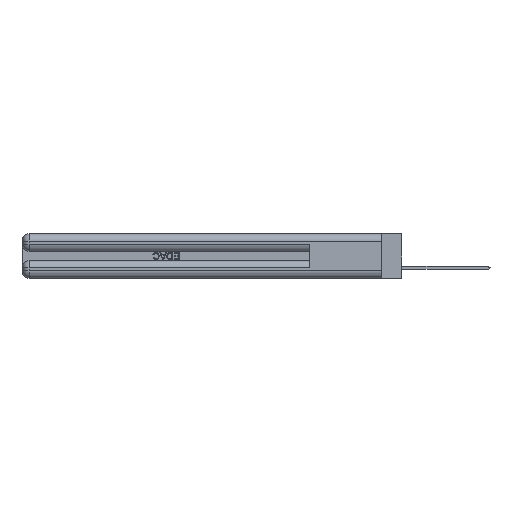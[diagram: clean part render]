
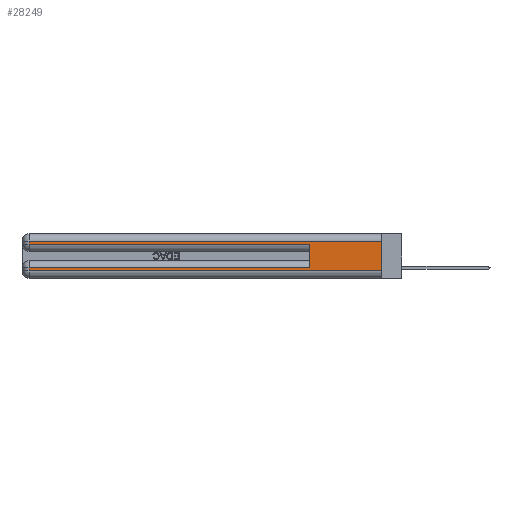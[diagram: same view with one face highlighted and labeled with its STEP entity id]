
A CAD part, left-side view. The second image highlights one B-rep face of the part: STEP entity #28249.
In plain terms, the highlighted planar face has unit normal (-1, 0, 0).
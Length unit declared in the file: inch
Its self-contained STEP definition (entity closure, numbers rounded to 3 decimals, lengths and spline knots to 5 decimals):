
#190 = LINE ( 'NONE', #8576, #42534 ) ;
#1328 = PLANE ( 'NONE',  #21933 ) ;
#1861 = DIRECTION ( 'NONE',  ( 0., 0., -1. ) ) ;
#3652 = CARTESIAN_POINT ( 'NONE',  ( 0., 2.94, 0.37 ) ) ;
#4363 = VECTOR ( 'NONE', #33084, 39.37008 ) ;
#4676 = VERTEX_POINT ( 'NONE', #18615 ) ;
#5362 = CARTESIAN_POINT ( 'NONE',  ( 0., 2.94, 0.37 ) ) ;
#5512 = CARTESIAN_POINT ( 'NONE',  ( 0., 0., 0.37 ) ) ;
#6326 = ORIENTED_EDGE ( 'NONE', *, *, #7794, .T. ) ;
#7229 = LINE ( 'NONE', #30174, #17976 ) ;
#7293 = DIRECTION ( 'NONE',  ( 0., -1., 0. ) ) ;
#7794 = EDGE_CURVE ( 'NONE', #32536, #46410, #32329, .T. ) ;
#8022 = EDGE_CURVE ( 'NONE', #26386, #9400, #7229, .T. ) ;
#8324 = EDGE_CURVE ( 'NONE', #19796, #9400, #21533, .T. ) ;
#8576 = CARTESIAN_POINT ( 'NONE',  ( 0., 0., 0.06 ) ) ;
#9400 = VERTEX_POINT ( 'NONE', #36453 ) ;
#9768 = ORIENTED_EDGE ( 'NONE', *, *, #26087, .T. ) ;
#9895 = VECTOR ( 'NONE', #1861, 39.37008 ) ;
#9980 = EDGE_LOOP ( 'NONE', ( #30056, #23095, #9768, #12261, #47401, #27262, #6326, #43001 ) ) ;
#10541 = CARTESIAN_POINT ( 'NONE',  ( 0., 0., 0.37 ) ) ;
#10996 = CARTESIAN_POINT ( 'NONE',  ( 0., 2.94, 0.06 ) ) ;
#12261 = ORIENTED_EDGE ( 'NONE', *, *, #8022, .T. ) ;
#13744 = CARTESIAN_POINT ( 'NONE',  ( 0., 0.6, 0.085 ) ) ;
#14297 = EDGE_CURVE ( 'NONE', #19796, #32536, #23885, .T. ) ;
#14438 = LINE ( 'NONE', #39794, #23378 ) ;
#17976 = VECTOR ( 'NONE', #7293, 39.37008 ) ;
#18615 = CARTESIAN_POINT ( 'NONE',  ( 0., 0., 0.06 ) ) ;
#19615 = CARTESIAN_POINT ( 'NONE',  ( 0., 0., 0.085 ) ) ;
#19714 = VECTOR ( 'NONE', #23392, 39.37008 ) ;
#19728 = VECTOR ( 'NONE', #23455, 39.37008 ) ;
#19796 = VERTEX_POINT ( 'NONE', #13744 ) ;
#21533 = LINE ( 'NONE', #46171, #19714 ) ;
#21619 = DIRECTION ( 'NONE',  ( 0., 1., 0. ) ) ;
#21933 = AXIS2_PLACEMENT_3D ( 'NONE', #5512, #31906, #39918 ) ;
#22198 = VECTOR ( 'NONE', #45498, 39.37008 ) ;
#23095 = ORIENTED_EDGE ( 'NONE', *, *, #29422, .T. ) ;
#23378 = VECTOR ( 'NONE', #21619, 39.37008 ) ;
#23392 = DIRECTION ( 'NONE',  ( 0., 0., 1. ) ) ;
#23455 = DIRECTION ( 'NONE',  ( 0., 1., 0. ) ) ;
#23595 = VERTEX_POINT ( 'NONE', #43406 ) ;
#23885 = LINE ( 'NONE', #19615, #19728 ) ;
#26087 = EDGE_CURVE ( 'NONE', #23595, #26386, #48061, .T. ) ;
#26386 = VERTEX_POINT ( 'NONE', #39602 ) ;
#27262 = ORIENTED_EDGE ( 'NONE', *, *, #14297, .T. ) ;
#28249 = ADVANCED_FACE ( 'NONE', ( #37315 ), #1328, .F. ) ;
#29422 = EDGE_CURVE ( 'NONE', #48343, #23595, #14438, .T. ) ;
#30056 = ORIENTED_EDGE ( 'NONE', *, *, #42595, .F. ) ;
#30174 = CARTESIAN_POINT ( 'NONE',  ( 0., 0., 0.285 ) ) ;
#30803 = CARTESIAN_POINT ( 'NONE',  ( 0., 2.94, 0.085 ) ) ;
#31906 = DIRECTION ( 'NONE',  ( 1., 0., 0. ) ) ;
#32329 = LINE ( 'NONE', #3652, #22198 ) ;
#32536 = VERTEX_POINT ( 'NONE', #30803 ) ;
#33084 = DIRECTION ( 'NONE',  ( 0., 0., -1. ) ) ;
#36453 = CARTESIAN_POINT ( 'NONE',  ( 0., 0.6, 0.285 ) ) ;
#37315 = FACE_OUTER_BOUND ( 'NONE', #9980, .T. ) ;
#38466 = CARTESIAN_POINT ( 'NONE',  ( 0., 0., 0.31 ) ) ;
#39602 = CARTESIAN_POINT ( 'NONE',  ( 0., 2.94, 0.285 ) ) ;
#39794 = CARTESIAN_POINT ( 'NONE',  ( 0., 0., 0.31 ) ) ;
#39918 = DIRECTION ( 'NONE',  ( 0., 0., -1. ) ) ;
#42534 = VECTOR ( 'NONE', #47076, 39.37008 ) ;
#42595 = EDGE_CURVE ( 'NONE', #48343, #4676, #44990, .T. ) ;
#43001 = ORIENTED_EDGE ( 'NONE', *, *, #47907, .T. ) ;
#43406 = CARTESIAN_POINT ( 'NONE',  ( 0., 2.94, 0.31 ) ) ;
#44990 = LINE ( 'NONE', #10541, #4363 ) ;
#45498 = DIRECTION ( 'NONE',  ( 0., 0., -1. ) ) ;
#46171 = CARTESIAN_POINT ( 'NONE',  ( 0., 0.6, 0.145 ) ) ;
#46410 = VERTEX_POINT ( 'NONE', #10996 ) ;
#47076 = DIRECTION ( 'NONE',  ( 0., -1., 0. ) ) ;
#47401 = ORIENTED_EDGE ( 'NONE', *, *, #8324, .F. ) ;
#47907 = EDGE_CURVE ( 'NONE', #46410, #4676, #190, .T. ) ;
#48061 = LINE ( 'NONE', #5362, #9895 ) ;
#48343 = VERTEX_POINT ( 'NONE', #38466 ) ;
